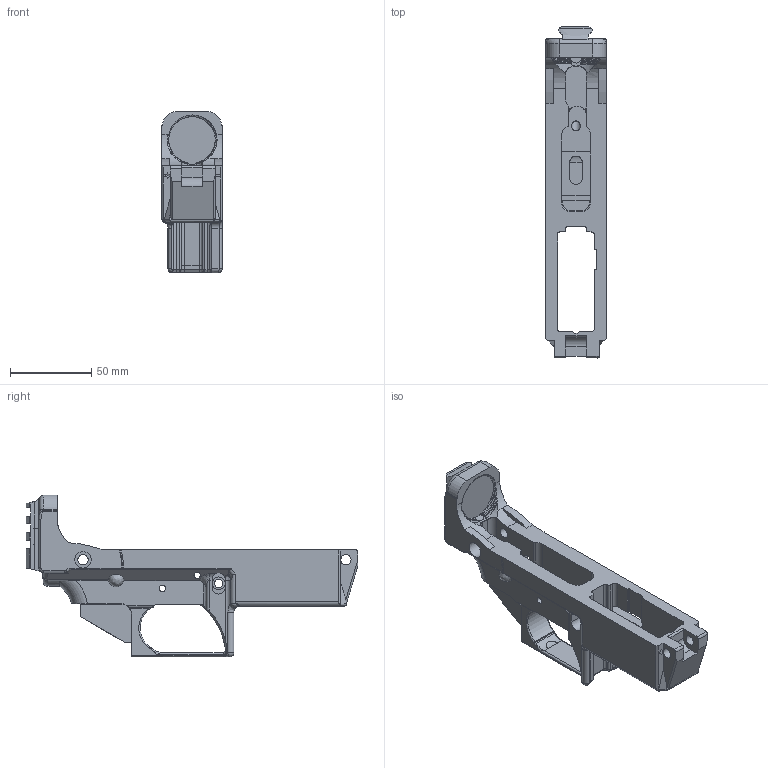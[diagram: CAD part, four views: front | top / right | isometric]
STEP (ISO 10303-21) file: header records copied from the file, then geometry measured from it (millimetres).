
FILE_DESCRIPTION(/* description */ (''),/* implementation_level */ '2;1');
FILE_NAME(/* name */ 'SG22 Lower Release v3.5.step',/* time_stamp */ '2021-08-05T20:23:42-07:00',/* author */ (''),/* organization */ (''),/* preprocessor_version */ 'ST-DEVELOPER v18.1',/* originating_system */ 'Autodesk Translation Framework v10.9.0.1377',/* authorisation */ '');
FILE_SCHEMA (('AUTOMOTIVE_DESIGN { 1 0 10303 214 3 1 1 }'));
Length unit declared in the file: millimetre
Products named in the file (1): SG22 Lower Release
Bounding box: 37.47 x 204.39 x 99.44 mm (x, y, z)
Surface area: 50978.6 mm2 (no closed solid volume)
Topology: 0 solids, 1 shells, 613 faces, 1713 edges, 1086 vertices
Faces by surface type: plane 233, cylinder 193, bspline 129, torus 33, cone 22, sphere 3
Full cylindrical faces by diameter (mm): 3.81 x1, 3.969 x4, 5.182 x1, 5.334 x1, 6.35 x4, 7.938 x1, 9.55 x2, 10.16 x1
Entity records: 28561 total; most frequent: CARTESIAN_POINT 13546, ORIENTED_EDGE 3409, DIRECTION 2787, EDGE_CURVE 1705, VERTEX_POINT 1086, AXIS2_PLACEMENT_3D 982, LINE 823, VECTOR 823
